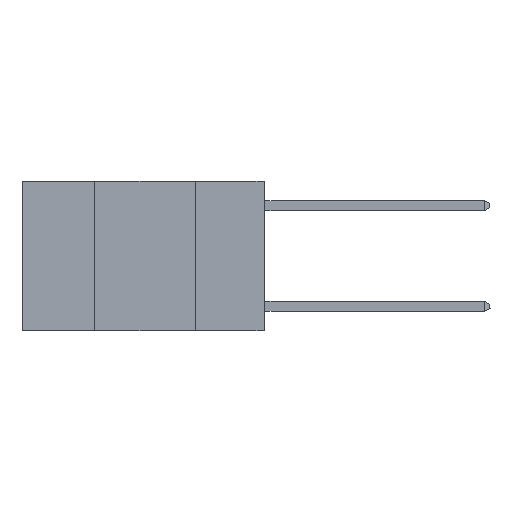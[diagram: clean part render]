
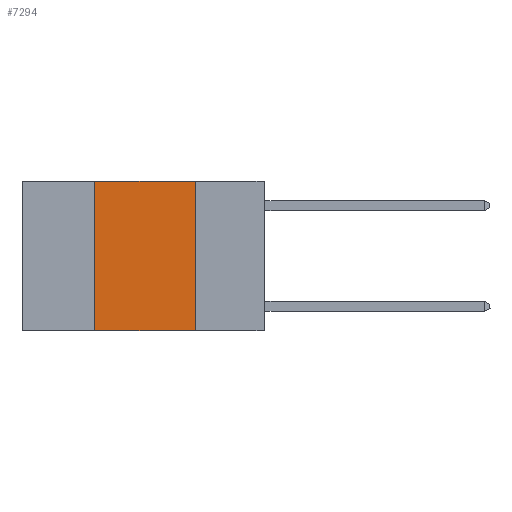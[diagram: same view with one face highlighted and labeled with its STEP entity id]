
A CAD part, left-side view. The second image highlights one B-rep face of the part: STEP entity #7294.
In plain terms, the highlighted planar face has unit normal (-1, 0, 0).
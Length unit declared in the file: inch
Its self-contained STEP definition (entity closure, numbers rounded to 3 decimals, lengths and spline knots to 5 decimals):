
#217 = EDGE_LOOP ( 'NONE', ( #11329, #7800, #7151, #5396 ) ) ;
#306 = VERTEX_POINT ( 'NONE', #7000 ) ;
#377 = VECTOR ( 'NONE', #10267, 39.37008 ) ;
#411 = CARTESIAN_POINT ( 'NONE',  ( 0., 0.42, 0. ) ) ;
#895 = CARTESIAN_POINT ( 'NONE',  ( 0., 0.17, 0. ) ) ;
#1038 = CARTESIAN_POINT ( 'NONE',  ( 0., 0.6, 0. ) ) ;
#1544 = FACE_OUTER_BOUND ( 'NONE', #217, .T. ) ;
#2467 = VECTOR ( 'NONE', #9139, 39.37008 ) ;
#2538 = VERTEX_POINT ( 'NONE', #411 ) ;
#2780 = CARTESIAN_POINT ( 'NONE',  ( 0., 0.6, -0.37 ) ) ;
#3135 = LINE ( 'NONE', #4909, #377 ) ;
#3583 = CARTESIAN_POINT ( 'NONE',  ( 0., 0.6, 0. ) ) ;
#3775 = VERTEX_POINT ( 'NONE', #11434 ) ;
#3861 = DIRECTION ( 'NONE',  ( 1., 0., 0. ) ) ;
#4738 = EDGE_CURVE ( 'NONE', #3775, #4851, #8454, .T. ) ;
#4851 = VERTEX_POINT ( 'NONE', #11023 ) ;
#4909 = CARTESIAN_POINT ( 'NONE',  ( 0., 0.42, 0. ) ) ;
#5133 = VECTOR ( 'NONE', #9008, 39.37008 ) ;
#5342 = EDGE_CURVE ( 'NONE', #306, #4851, #9680, .T. ) ;
#5396 = ORIENTED_EDGE ( 'NONE', *, *, #5342, .T. ) ;
#6041 = VECTOR ( 'NONE', #8208, 39.37008 ) ;
#7000 = CARTESIAN_POINT ( 'NONE',  ( 0., 0.42, -0.37 ) ) ;
#7151 = ORIENTED_EDGE ( 'NONE', *, *, #7377, .F. ) ;
#7294 = ADVANCED_FACE ( 'NONE', ( #1544 ), #10105, .F. ) ;
#7377 = EDGE_CURVE ( 'NONE', #306, #2538, #3135, .T. ) ;
#7608 = EDGE_CURVE ( 'NONE', #2538, #3775, #9625, .T. ) ;
#7800 = ORIENTED_EDGE ( 'NONE', *, *, #7608, .F. ) ;
#8208 = DIRECTION ( 'NONE',  ( 0., 0., -1. ) ) ;
#8454 = LINE ( 'NONE', #895, #6041 ) ;
#9008 = DIRECTION ( 'NONE',  ( 0., -1., 0. ) ) ;
#9116 = AXIS2_PLACEMENT_3D ( 'NONE', #1038, #3861, #10149 ) ;
#9139 = DIRECTION ( 'NONE',  ( 0., -1., 0. ) ) ;
#9625 = LINE ( 'NONE', #3583, #5133 ) ;
#9680 = LINE ( 'NONE', #2780, #2467 ) ;
#10105 = PLANE ( 'NONE',  #9116 ) ;
#10149 = DIRECTION ( 'NONE',  ( 0., 0., -1. ) ) ;
#10267 = DIRECTION ( 'NONE',  ( 0., 0., 1. ) ) ;
#11023 = CARTESIAN_POINT ( 'NONE',  ( 0., 0.17, -0.37 ) ) ;
#11329 = ORIENTED_EDGE ( 'NONE', *, *, #4738, .F. ) ;
#11434 = CARTESIAN_POINT ( 'NONE',  ( 0., 0.17, 0. ) ) ;
